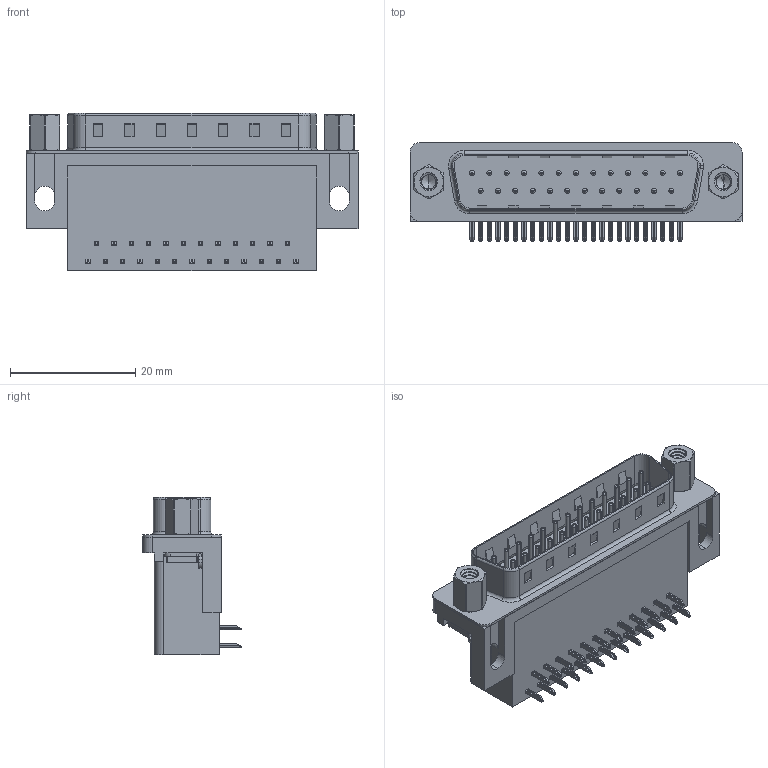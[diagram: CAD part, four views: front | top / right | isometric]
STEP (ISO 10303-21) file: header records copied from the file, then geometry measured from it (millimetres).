
FILE_DESCRIPTION (( 'STEP AP203' ), '1' );
FILE_NAME ('625-025-362-503.STEP', '2018-11-06T02:37:25', ( '' ), ( '' ), 'SwSTEP 2.0', 'SolidWorks 2016', '' );
FILE_SCHEMA (( 'CONFIG_CONTROL_DESIGN' ));
Length unit declared in the file: millimetre
Products named in the file (8): 625-025-362-503; 625 Housing_25 Socket; 625 Shell_25 Socket; 625 Contact Bottom; 625 Contact Top; 625 Non Board Mount; 625 4-40 Threaded Rivet; 625 4-40 Hex Standoff 5
Assembly tree (33 placements, depth 2):
  625-025-362-503
    625 Housing_25 Socket
    625 Shell_25 Socket
    625 Contact Bottom  x12
    625 Contact Top  x13
    625 Non Board Mount  x2
    625 4-40 Threaded Rivet  x2
    625 4-40 Hex Standoff 5  x2
Bounding box: 53.04 x 15.73 x 25.16 mm (x, y, z)
Volume: 9350.1 mm3; surface area: 9210.5 mm2
Topology: 33 solids, 33 shells, 2389 faces, 5955 edges, 3689 vertices
Faces by surface type: plane 1429, cylinder 729, torus 181, cone 32, bspline 18
Entity records: 27420 total; most frequent: CARTESIAN_POINT 8414, DIRECTION 3629, ORIENTED_EDGE 3616, EDGE_CURVE 1808, AXIS2_PLACEMENT_3D 1212, VECTOR 1205, LINE 1205, VERTEX_POINT 1162
